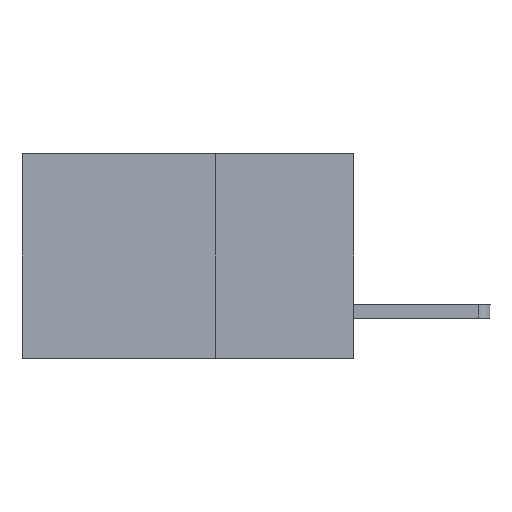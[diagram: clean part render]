
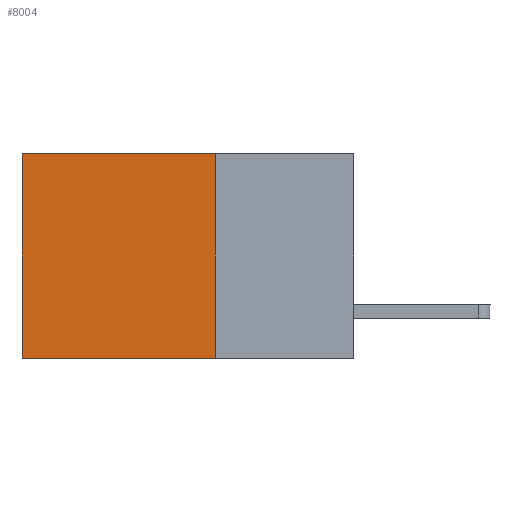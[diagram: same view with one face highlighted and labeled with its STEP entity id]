
A CAD part, left-side view. The second image highlights one B-rep face of the part: STEP entity #8004.
In plain terms, the highlighted planar face has unit normal (-1, 0, 0).
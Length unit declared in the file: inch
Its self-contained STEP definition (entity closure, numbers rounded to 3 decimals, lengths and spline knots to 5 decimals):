
#484 = VECTOR ( 'NONE', #6988, 39.37008 ) ;
#765 = EDGE_CURVE ( 'NONE', #3996, #5916, #7588, .T. ) ;
#767 = AXIS2_PLACEMENT_3D ( 'NONE', #1631, #3651, #2879 ) ;
#938 = EDGE_LOOP ( 'NONE', ( #5486, #5558, #1172, #5357 ) ) ;
#1086 = VECTOR ( 'NONE', #7829, 39.37008 ) ;
#1172 = ORIENTED_EDGE ( 'NONE', *, *, #765, .F. ) ;
#1220 = VECTOR ( 'NONE', #6856, 39.37008 ) ;
#1447 = DIRECTION ( 'NONE',  ( 0., 0., -1. ) ) ;
#1469 = CARTESIAN_POINT ( 'NONE',  ( 0.2875, 0.25, -0.37 ) ) ;
#1631 = CARTESIAN_POINT ( 'NONE',  ( 0.2875, 0.25, 0. ) ) ;
#2182 = FACE_OUTER_BOUND ( 'NONE', #938, .T. ) ;
#2402 = CARTESIAN_POINT ( 'NONE',  ( 0.2875, 0.6, -0.37 ) ) ;
#2879 = DIRECTION ( 'NONE',  ( 0., 0., -1. ) ) ;
#3463 = VERTEX_POINT ( 'NONE', #5408 ) ;
#3600 = PLANE ( 'NONE',  #767 ) ;
#3651 = DIRECTION ( 'NONE',  ( 1., 0., 0. ) ) ;
#3925 = CARTESIAN_POINT ( 'NONE',  ( 0.2875, 0.25, 0. ) ) ;
#3996 = VERTEX_POINT ( 'NONE', #7808 ) ;
#4195 = EDGE_CURVE ( 'NONE', #3463, #7022, #7638, .T. ) ;
#5357 = ORIENTED_EDGE ( 'NONE', *, *, #8048, .T. ) ;
#5408 = CARTESIAN_POINT ( 'NONE',  ( 0.2875, 0.6, 0. ) ) ;
#5445 = CARTESIAN_POINT ( 'NONE',  ( 0.2875, 0.6, 0. ) ) ;
#5486 = ORIENTED_EDGE ( 'NONE', *, *, #4195, .T. ) ;
#5558 = ORIENTED_EDGE ( 'NONE', *, *, #7978, .F. ) ;
#5916 = VERTEX_POINT ( 'NONE', #7905 ) ;
#6856 = DIRECTION ( 'NONE',  ( 0., 1., 0. ) ) ;
#6932 = CARTESIAN_POINT ( 'NONE',  ( 0.2875, 0.25, 0. ) ) ;
#6988 = DIRECTION ( 'NONE',  ( 0., 1., 0. ) ) ;
#7022 = VERTEX_POINT ( 'NONE', #2402 ) ;
#7588 = LINE ( 'NONE', #3925, #1086 ) ;
#7638 = LINE ( 'NONE', #5445, #8157 ) ;
#7808 = CARTESIAN_POINT ( 'NONE',  ( 0.2875, 0.25, 0. ) ) ;
#7829 = DIRECTION ( 'NONE',  ( 0., 0., -1. ) ) ;
#7905 = CARTESIAN_POINT ( 'NONE',  ( 0.2875, 0.25, -0.37 ) ) ;
#7927 = LINE ( 'NONE', #1469, #1220 ) ;
#7978 = EDGE_CURVE ( 'NONE', #5916, #7022, #7927, .T. ) ;
#8004 = ADVANCED_FACE ( 'NONE', ( #2182 ), #3600, .F. ) ;
#8048 = EDGE_CURVE ( 'NONE', #3996, #3463, #8344, .T. ) ;
#8157 = VECTOR ( 'NONE', #1447, 39.37008 ) ;
#8344 = LINE ( 'NONE', #6932, #484 ) ;
